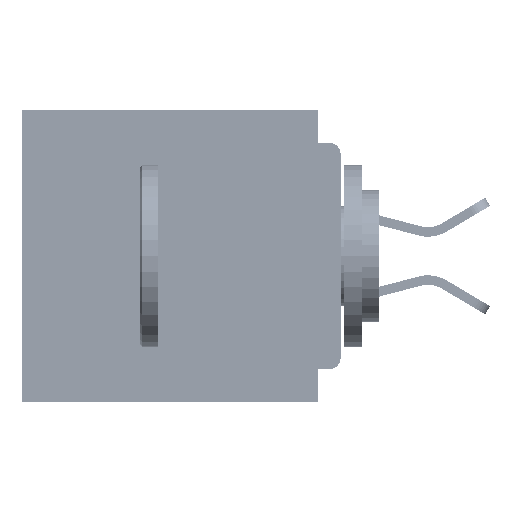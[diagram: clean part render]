
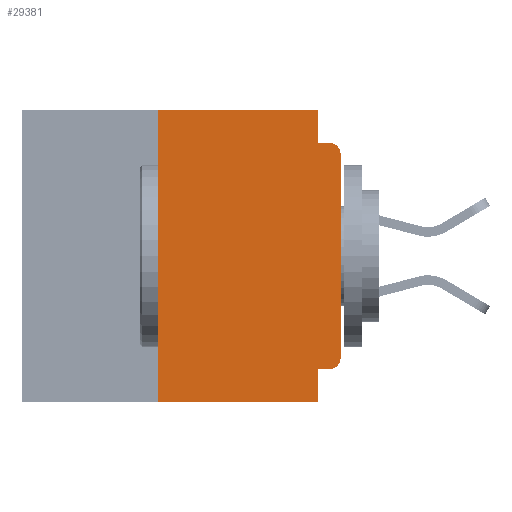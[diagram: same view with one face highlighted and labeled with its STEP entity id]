
A CAD part, left-side view. The second image highlights one B-rep face of the part: STEP entity #29381.
In plain terms, the highlighted planar face has unit normal (-1, 0, 0).
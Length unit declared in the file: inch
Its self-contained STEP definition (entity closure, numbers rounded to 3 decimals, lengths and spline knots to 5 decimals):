
#126 = DIRECTION ( 'NONE',  ( -1., 0., 0. ) ) ;
#2044 = AXIS2_PLACEMENT_3D ( 'NONE', #35078, #7802, #39621 ) ;
#2085 = ORIENTED_EDGE ( 'NONE', *, *, #10283, .F. ) ;
#2208 = VERTEX_POINT ( 'NONE', #36959 ) ;
#2377 = VECTOR ( 'NONE', #28664, 39.37008 ) ;
#2635 = EDGE_CURVE ( 'NONE', #2208, #32547, #33520, .T. ) ;
#3220 = AXIS2_PLACEMENT_3D ( 'NONE', #6967, #52455, #25328 ) ;
#3798 = CARTESIAN_POINT ( 'NONE',  ( 0., 0.25, -0.4 ) ) ;
#4901 = DIRECTION ( 'NONE',  ( 0., -1., 0. ) ) ;
#5925 = DIRECTION ( 'NONE',  ( 0., -1., 0. ) ) ;
#6669 = VECTOR ( 'NONE', #18664, 39.37008 ) ;
#6967 = CARTESIAN_POINT ( 'NONE',  ( 0., 0.437, 0. ) ) ;
#7802 = DIRECTION ( 'NONE',  ( -1., 0., 0. ) ) ;
#7837 = VERTEX_POINT ( 'NONE', #54660 ) ;
#10283 = EDGE_CURVE ( 'NONE', #54800, #26765, #16500, .T. ) ;
#11447 = AXIS2_PLACEMENT_3D ( 'NONE', #27400, #126, #31930 ) ;
#11802 = EDGE_CURVE ( 'NONE', #44760, #54800, #54007, .T. ) ;
#12044 = CARTESIAN_POINT ( 'NONE',  ( 0., 0.015, -0.045 ) ) ;
#13544 = CARTESIAN_POINT ( 'NONE',  ( 0., 0.25, 0. ) ) ;
#14097 = CARTESIAN_POINT ( 'NONE',  ( 0., 0.25, -0.4 ) ) ;
#14112 = ORIENTED_EDGE ( 'NONE', *, *, #42954, .T. ) ;
#15127 = CIRCLE ( 'NONE', #2044, 0.015 ) ;
#15825 = CIRCLE ( 'NONE', #11447, 0.015 ) ;
#15864 = DIRECTION ( 'NONE',  ( 0., -1., 0. ) ) ;
#16500 = LINE ( 'NONE', #54762, #39213 ) ;
#18219 = ORIENTED_EDGE ( 'NONE', *, *, #57225, .F. ) ;
#18613 = VERTEX_POINT ( 'NONE', #26033 ) ;
#18664 = DIRECTION ( 'NONE',  ( 0., 0., -1. ) ) ;
#18819 = LINE ( 'NONE', #36716, #6669 ) ;
#19063 = VECTOR ( 'NONE', #57633, 39.37008 ) ;
#20628 = VERTEX_POINT ( 'NONE', #47672 ) ;
#21046 = LINE ( 'NONE', #43070, #43765 ) ;
#24014 = EDGE_CURVE ( 'NONE', #26879, #18613, #53838, .T. ) ;
#25328 = DIRECTION ( 'NONE',  ( 0., 0., -1. ) ) ;
#25953 = CARTESIAN_POINT ( 'NONE',  ( 0., 0., 0. ) ) ;
#26033 = CARTESIAN_POINT ( 'NONE',  ( 0., 0., -0.06 ) ) ;
#26255 = ORIENTED_EDGE ( 'NONE', *, *, #24014, .T. ) ;
#26765 = VERTEX_POINT ( 'NONE', #30766 ) ;
#26879 = VERTEX_POINT ( 'NONE', #31719 ) ;
#27400 = CARTESIAN_POINT ( 'NONE',  ( 0., 0.015, -0.34 ) ) ;
#28664 = DIRECTION ( 'NONE',  ( 0., 1., 0. ) ) ;
#29381 = ADVANCED_FACE ( 'NONE', ( #30960 ), #47911, .F. ) ;
#30503 = VECTOR ( 'NONE', #54362, 39.37008 ) ;
#30766 = CARTESIAN_POINT ( 'NONE',  ( 0., 0.031, 0. ) ) ;
#30960 = FACE_OUTER_BOUND ( 'NONE', #38037, .T. ) ;
#31287 = VERTEX_POINT ( 'NONE', #53839 ) ;
#31555 = CARTESIAN_POINT ( 'NONE',  ( 0., 0.031, 0. ) ) ;
#31719 = CARTESIAN_POINT ( 'NONE',  ( 0., 0., -0.34 ) ) ;
#31930 = DIRECTION ( 'NONE',  ( 0., 0., -1. ) ) ;
#32547 = VERTEX_POINT ( 'NONE', #12044 ) ;
#33520 = LINE ( 'NONE', #37747, #57603 ) ;
#35078 = CARTESIAN_POINT ( 'NONE',  ( 0., 0.015, -0.06 ) ) ;
#36716 = CARTESIAN_POINT ( 'NONE',  ( 0., 0.031, -0.4 ) ) ;
#36959 = CARTESIAN_POINT ( 'NONE',  ( 0., 0.031, -0.045 ) ) ;
#37747 = CARTESIAN_POINT ( 'NONE',  ( 0., 0., -0.045 ) ) ;
#38037 = EDGE_LOOP ( 'NONE', ( #26255, #54684, #46964, #18219, #2085, #52396, #46265, #43832, #47237, #14112 ) ) ;
#39213 = VECTOR ( 'NONE', #4901, 39.37008 ) ;
#39621 = DIRECTION ( 'NONE',  ( 0., 0., -1. ) ) ;
#40065 = LINE ( 'NONE', #42137, #2377 ) ;
#42137 = CARTESIAN_POINT ( 'NONE',  ( 0., 0., -0.355 ) ) ;
#42587 = LINE ( 'NONE', #31555, #30503 ) ;
#42954 = EDGE_CURVE ( 'NONE', #31287, #26879, #15825, .T. ) ;
#43070 = CARTESIAN_POINT ( 'NONE',  ( 0., 0.437, -0.4 ) ) ;
#43765 = VECTOR ( 'NONE', #15864, 39.37008 ) ;
#43832 = ORIENTED_EDGE ( 'NONE', *, *, #48972, .F. ) ;
#44760 = VERTEX_POINT ( 'NONE', #14097 ) ;
#46265 = ORIENTED_EDGE ( 'NONE', *, *, #53418, .T. ) ;
#46964 = ORIENTED_EDGE ( 'NONE', *, *, #2635, .F. ) ;
#47237 = ORIENTED_EDGE ( 'NONE', *, *, #54553, .F. ) ;
#47672 = CARTESIAN_POINT ( 'NONE',  ( 0., 0.031, -0.4 ) ) ;
#47911 = PLANE ( 'NONE',  #3220 ) ;
#48972 = EDGE_CURVE ( 'NONE', #7837, #20628, #18819, .T. ) ;
#49093 = DIRECTION ( 'NONE',  ( 0., 0., 1. ) ) ;
#52396 = ORIENTED_EDGE ( 'NONE', *, *, #11802, .F. ) ;
#52455 = DIRECTION ( 'NONE',  ( 1., 0., 0. ) ) ;
#53418 = EDGE_CURVE ( 'NONE', #44760, #20628, #21046, .T. ) ;
#53838 = LINE ( 'NONE', #25953, #19063 ) ;
#53839 = CARTESIAN_POINT ( 'NONE',  ( 0., 0.015, -0.355 ) ) ;
#54007 = LINE ( 'NONE', #3798, #55419 ) ;
#54362 = DIRECTION ( 'NONE',  ( 0., 0., -1. ) ) ;
#54553 = EDGE_CURVE ( 'NONE', #31287, #7837, #40065, .T. ) ;
#54660 = CARTESIAN_POINT ( 'NONE',  ( 0., 0.031, -0.355 ) ) ;
#54684 = ORIENTED_EDGE ( 'NONE', *, *, #55934, .T. ) ;
#54762 = CARTESIAN_POINT ( 'NONE',  ( 0., 0.437, 0. ) ) ;
#54800 = VERTEX_POINT ( 'NONE', #13544 ) ;
#55419 = VECTOR ( 'NONE', #49093, 39.37008 ) ;
#55934 = EDGE_CURVE ( 'NONE', #18613, #32547, #15127, .T. ) ;
#57225 = EDGE_CURVE ( 'NONE', #26765, #2208, #42587, .T. ) ;
#57603 = VECTOR ( 'NONE', #5925, 39.37008 ) ;
#57633 = DIRECTION ( 'NONE',  ( 0., 0., 1. ) ) ;
